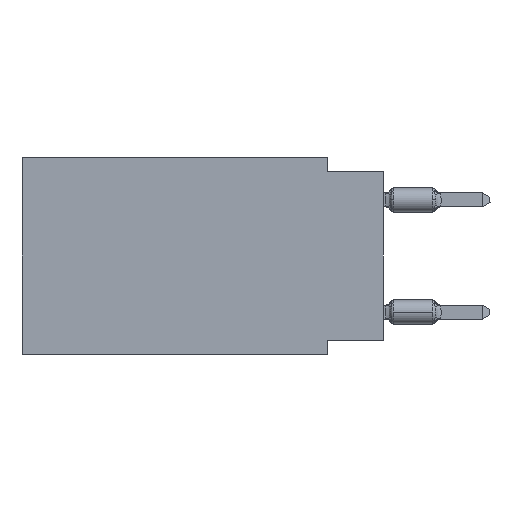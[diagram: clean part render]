
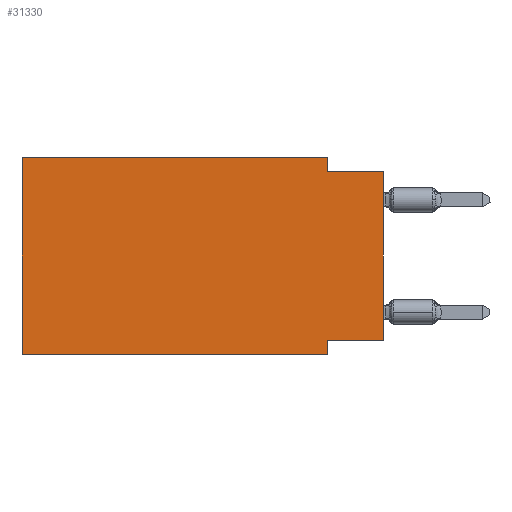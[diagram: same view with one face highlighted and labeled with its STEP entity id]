
A CAD part, left-side view. The second image highlights one B-rep face of the part: STEP entity #31330.
In plain terms, the highlighted planar face has unit normal (-1, 0, 0).
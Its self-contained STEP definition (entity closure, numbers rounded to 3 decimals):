
#234 = DIRECTION ( 'NONE',  ( 0., -1., 0. ) ) ;
#320 = VECTOR ( 'NONE', #18194, 1000. ) ;
#836 = VERTEX_POINT ( 'NONE', #25857 ) ;
#1645 = EDGE_CURVE ( 'NONE', #836, #8951, #27759, .T. ) ;
#1767 = VERTEX_POINT ( 'NONE', #31716 ) ;
#1976 = VECTOR ( 'NONE', #28178, 1000. ) ;
#2255 = ORIENTED_EDGE ( 'NONE', *, *, #17416, .F. ) ;
#2715 = EDGE_CURVE ( 'NONE', #19983, #34793, #4802, .T. ) ;
#2725 = DIRECTION ( 'NONE',  ( 0., 0., -1. ) ) ;
#4214 = ORIENTED_EDGE ( 'NONE', *, *, #21443, .T. ) ;
#4802 = LINE ( 'NONE', #27051, #320 ) ;
#5477 = ORIENTED_EDGE ( 'NONE', *, *, #19818, .F. ) ;
#5784 = CARTESIAN_POINT ( 'NONE',  ( 0., 16.383, 0. ) ) ;
#6106 = CARTESIAN_POINT ( 'NONE',  ( 0., 0., -0.635 ) ) ;
#8120 = CARTESIAN_POINT ( 'NONE',  ( 0., 0., 0. ) ) ;
#8159 = CARTESIAN_POINT ( 'NONE',  ( 0., 2.54, -0.635 ) ) ;
#8186 = ORIENTED_EDGE ( 'NONE', *, *, #1645, .F. ) ;
#8677 = ORIENTED_EDGE ( 'NONE', *, *, #34806, .F. ) ;
#8951 = VERTEX_POINT ( 'NONE', #8159 ) ;
#9000 = LINE ( 'NONE', #6106, #1976 ) ;
#9070 = ORIENTED_EDGE ( 'NONE', *, *, #2715, .F. ) ;
#10379 = VERTEX_POINT ( 'NONE', #29480 ) ;
#10842 = PLANE ( 'NONE',  #16588 ) ;
#10868 = LINE ( 'NONE', #34935, #33873 ) ;
#11823 = CARTESIAN_POINT ( 'NONE',  ( 0., 2.54, 0. ) ) ;
#12892 = VERTEX_POINT ( 'NONE', #32285 ) ;
#13580 = DIRECTION ( 'NONE',  ( 0., 1., 0. ) ) ;
#14110 = EDGE_LOOP ( 'NONE', ( #4214, #2255, #8186, #8677, #32378, #19134, #9070, #5477 ) ) ;
#14819 = LINE ( 'NONE', #26033, #32772 ) ;
#15822 = VECTOR ( 'NONE', #25379, 1000. ) ;
#15853 = VERTEX_POINT ( 'NONE', #33624 ) ;
#16588 = AXIS2_PLACEMENT_3D ( 'NONE', #5784, #16636, #2725 ) ;
#16636 = DIRECTION ( 'NONE',  ( 1., 0., 0. ) ) ;
#17045 = CARTESIAN_POINT ( 'NONE',  ( 0., 16.383, 0. ) ) ;
#17355 = DIRECTION ( 'NONE',  ( 0., 0., 1. ) ) ;
#17416 = EDGE_CURVE ( 'NONE', #8951, #1767, #9000, .T. ) ;
#18194 = DIRECTION ( 'NONE',  ( 0., 0., -1. ) ) ;
#19134 = ORIENTED_EDGE ( 'NONE', *, *, #20800, .T. ) ;
#19818 = EDGE_CURVE ( 'NONE', #12892, #19983, #10868, .T. ) ;
#19983 = VERTEX_POINT ( 'NONE', #33828 ) ;
#20142 = CARTESIAN_POINT ( 'NONE',  ( 0., 16.383, -8.89 ) ) ;
#20800 = EDGE_CURVE ( 'NONE', #10379, #34793, #22301, .T. ) ;
#21443 = EDGE_CURVE ( 'NONE', #12892, #1767, #32902, .T. ) ;
#22231 = FACE_OUTER_BOUND ( 'NONE', #14110, .T. ) ;
#22290 = VECTOR ( 'NONE', #32372, 1000. ) ;
#22301 = LINE ( 'NONE', #20142, #28059 ) ;
#23191 = CARTESIAN_POINT ( 'NONE',  ( 0., 2.54, -8.89 ) ) ;
#25379 = DIRECTION ( 'NONE',  ( 0., -1., 0. ) ) ;
#25762 = DIRECTION ( 'NONE',  ( 0., 0., -1. ) ) ;
#25857 = CARTESIAN_POINT ( 'NONE',  ( 0., 2.54, 0. ) ) ;
#26033 = CARTESIAN_POINT ( 'NONE',  ( 0., 16.383, 0. ) ) ;
#26846 = VECTOR ( 'NONE', #25762, 1000. ) ;
#27051 = CARTESIAN_POINT ( 'NONE',  ( 0., 2.54, -8.89 ) ) ;
#27759 = LINE ( 'NONE', #11823, #26846 ) ;
#28059 = VECTOR ( 'NONE', #234, 1000. ) ;
#28178 = DIRECTION ( 'NONE',  ( 0., -1., 0. ) ) ;
#29480 = CARTESIAN_POINT ( 'NONE',  ( 0., 16.383, -8.89 ) ) ;
#30614 = LINE ( 'NONE', #17045, #15822 ) ;
#31330 = ADVANCED_FACE ( 'NONE', ( #22231 ), #10842, .F. ) ;
#31444 = EDGE_CURVE ( 'NONE', #10379, #15853, #14819, .T. ) ;
#31716 = CARTESIAN_POINT ( 'NONE',  ( 0., 0., -0.635 ) ) ;
#32285 = CARTESIAN_POINT ( 'NONE',  ( 0., 0., -8.255 ) ) ;
#32372 = DIRECTION ( 'NONE',  ( 0., 0., 1. ) ) ;
#32378 = ORIENTED_EDGE ( 'NONE', *, *, #31444, .F. ) ;
#32772 = VECTOR ( 'NONE', #17355, 1000. ) ;
#32902 = LINE ( 'NONE', #8120, #22290 ) ;
#33624 = CARTESIAN_POINT ( 'NONE',  ( 0., 16.383, 0. ) ) ;
#33828 = CARTESIAN_POINT ( 'NONE',  ( 0., 2.54, -8.255 ) ) ;
#33873 = VECTOR ( 'NONE', #13580, 1000. ) ;
#34793 = VERTEX_POINT ( 'NONE', #23191 ) ;
#34806 = EDGE_CURVE ( 'NONE', #15853, #836, #30614, .T. ) ;
#34935 = CARTESIAN_POINT ( 'NONE',  ( 0., 0., -8.255 ) ) ;
